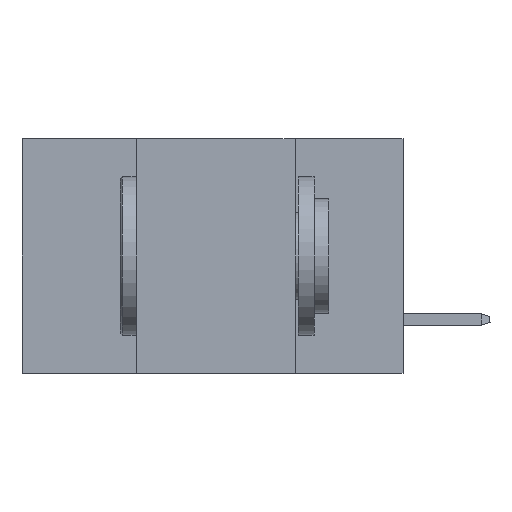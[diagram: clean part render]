
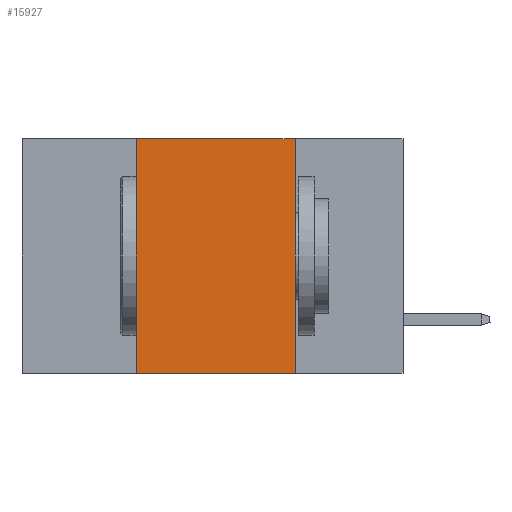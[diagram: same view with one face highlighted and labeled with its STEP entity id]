
A CAD part, left-side view. The second image highlights one B-rep face of the part: STEP entity #15927.
In plain terms, the highlighted planar face has unit normal (-1, 0, 0).
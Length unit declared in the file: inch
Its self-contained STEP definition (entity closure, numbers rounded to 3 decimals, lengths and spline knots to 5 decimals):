
#595 = CARTESIAN_POINT ( 'NONE',  ( 0., 0.6, -0.37 ) ) ;
#784 = CARTESIAN_POINT ( 'NONE',  ( 0., 0.17, 0. ) ) ;
#1752 = ORIENTED_EDGE ( 'NONE', *, *, #5616, .F. ) ;
#1794 = FACE_OUTER_BOUND ( 'NONE', #18065, .T. ) ;
#2039 = ORIENTED_EDGE ( 'NONE', *, *, #10265, .T. ) ;
#2135 = VERTEX_POINT ( 'NONE', #9403 ) ;
#3143 = CARTESIAN_POINT ( 'NONE',  ( 0., 0.6, 0. ) ) ;
#3374 = DIRECTION ( 'NONE',  ( 0., 0., -1. ) ) ;
#4901 = DIRECTION ( 'NONE',  ( 0., -1., 0. ) ) ;
#5323 = DIRECTION ( 'NONE',  ( 1., 0., 0. ) ) ;
#5616 = EDGE_CURVE ( 'NONE', #18592, #13047, #7700, .T. ) ;
#6086 = CARTESIAN_POINT ( 'NONE',  ( 0., 0.42, 0. ) ) ;
#7700 = LINE ( 'NONE', #14261, #16466 ) ;
#7910 = CARTESIAN_POINT ( 'NONE',  ( 0., 0.17, -0.37 ) ) ;
#8225 = CARTESIAN_POINT ( 'NONE',  ( 0., 0.42, -0.37 ) ) ;
#8380 = EDGE_CURVE ( 'NONE', #2135, #18592, #13589, .T. ) ;
#8814 = VECTOR ( 'NONE', #13066, 39.37008 ) ;
#9390 = DIRECTION ( 'NONE',  ( 0., -1., 0. ) ) ;
#9403 = CARTESIAN_POINT ( 'NONE',  ( 0., 0.42, 0. ) ) ;
#9422 = LINE ( 'NONE', #6086, #8814 ) ;
#10265 = EDGE_CURVE ( 'NONE', #11762, #13047, #12594, .T. ) ;
#11762 = VERTEX_POINT ( 'NONE', #8225 ) ;
#12594 = LINE ( 'NONE', #595, #13287 ) ;
#13040 = AXIS2_PLACEMENT_3D ( 'NONE', #3143, #5323, #3374 ) ;
#13047 = VERTEX_POINT ( 'NONE', #7910 ) ;
#13066 = DIRECTION ( 'NONE',  ( 0., 0., 1. ) ) ;
#13268 = VECTOR ( 'NONE', #4901, 39.37008 ) ;
#13287 = VECTOR ( 'NONE', #9390, 39.37008 ) ;
#13589 = LINE ( 'NONE', #18744, #13268 ) ;
#14016 = PLANE ( 'NONE',  #13040 ) ;
#14261 = CARTESIAN_POINT ( 'NONE',  ( 0., 0.17, 0. ) ) ;
#15927 = ADVANCED_FACE ( 'NONE', ( #1794 ), #14016, .F. ) ;
#16203 = DIRECTION ( 'NONE',  ( 0., 0., -1. ) ) ;
#16466 = VECTOR ( 'NONE', #16203, 39.37008 ) ;
#18033 = ORIENTED_EDGE ( 'NONE', *, *, #8380, .F. ) ;
#18065 = EDGE_LOOP ( 'NONE', ( #1752, #18033, #18774, #2039 ) ) ;
#18592 = VERTEX_POINT ( 'NONE', #784 ) ;
#18744 = CARTESIAN_POINT ( 'NONE',  ( 0., 0.6, 0. ) ) ;
#18774 = ORIENTED_EDGE ( 'NONE', *, *, #21878, .F. ) ;
#21878 = EDGE_CURVE ( 'NONE', #11762, #2135, #9422, .T. ) ;
